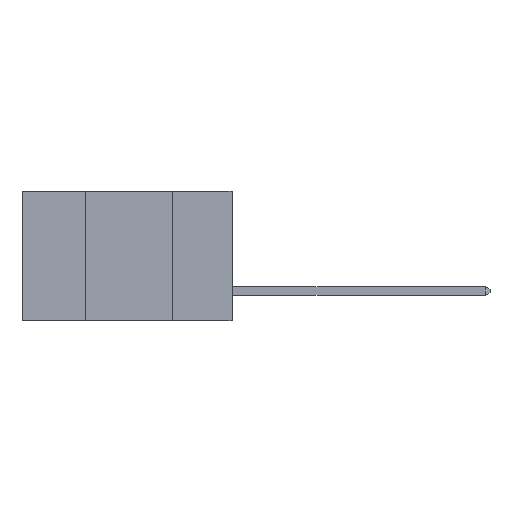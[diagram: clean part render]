
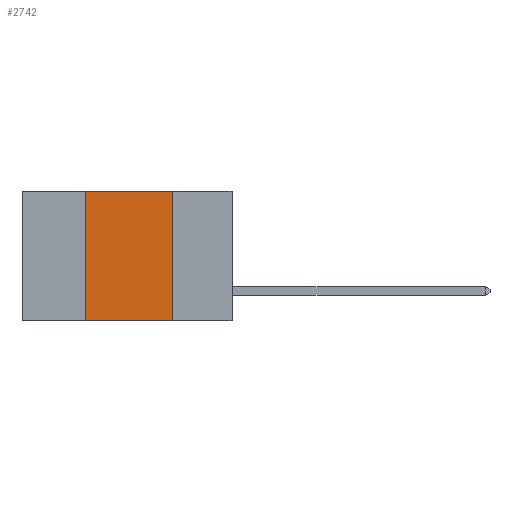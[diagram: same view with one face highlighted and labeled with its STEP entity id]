
A CAD part, left-side view. The second image highlights one B-rep face of the part: STEP entity #2742.
In plain terms, the highlighted planar face has unit normal (-1, 0, 0).
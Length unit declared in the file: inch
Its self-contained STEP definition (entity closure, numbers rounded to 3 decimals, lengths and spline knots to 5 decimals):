
#84 = DIRECTION ( 'NONE',  ( 0., -1., 0. ) ) ;
#383 = ORIENTED_EDGE ( 'NONE', *, *, #1739, .F. ) ;
#463 = VERTEX_POINT ( 'NONE', #9577 ) ;
#886 = VERTEX_POINT ( 'NONE', #2946 ) ;
#1046 = CARTESIAN_POINT ( 'NONE',  ( 0., 0.17, 0. ) ) ;
#1118 = DIRECTION ( 'NONE',  ( 0., 0., 1. ) ) ;
#1592 = AXIS2_PLACEMENT_3D ( 'NONE', #8293, #4157, #11375 ) ;
#1739 = EDGE_CURVE ( 'NONE', #463, #2903, #11052, .T. ) ;
#2147 = DIRECTION ( 'NONE',  ( 0., 0., -1. ) ) ;
#2742 = ADVANCED_FACE ( 'NONE', ( #7658 ), #12336, .F. ) ;
#2903 = VERTEX_POINT ( 'NONE', #6084 ) ;
#2946 = CARTESIAN_POINT ( 'NONE',  ( 0., 0.17, -0.37 ) ) ;
#3523 = CARTESIAN_POINT ( 'NONE',  ( 0., 0.42, -0.37 ) ) ;
#3797 = ORIENTED_EDGE ( 'NONE', *, *, #4467, .F. ) ;
#3812 = LINE ( 'NONE', #10682, #6924 ) ;
#4157 = DIRECTION ( 'NONE',  ( 1., 0., 0. ) ) ;
#4366 = CARTESIAN_POINT ( 'NONE',  ( 0., 0.42, 0. ) ) ;
#4467 = EDGE_CURVE ( 'NONE', #2903, #886, #12710, .T. ) ;
#5779 = DIRECTION ( 'NONE',  ( 0., -1., 0. ) ) ;
#5930 = EDGE_CURVE ( 'NONE', #6036, #886, #3812, .T. ) ;
#6036 = VERTEX_POINT ( 'NONE', #3523 ) ;
#6084 = CARTESIAN_POINT ( 'NONE',  ( 0., 0.17, 0. ) ) ;
#6924 = VECTOR ( 'NONE', #84, 39.37008 ) ;
#7294 = EDGE_LOOP ( 'NONE', ( #3797, #383, #13451, #9332 ) ) ;
#7658 = FACE_OUTER_BOUND ( 'NONE', #7294, .T. ) ;
#8064 = EDGE_CURVE ( 'NONE', #6036, #463, #11810, .T. ) ;
#8293 = CARTESIAN_POINT ( 'NONE',  ( 0., 0.6, 0. ) ) ;
#9090 = VECTOR ( 'NONE', #1118, 39.37008 ) ;
#9332 = ORIENTED_EDGE ( 'NONE', *, *, #5930, .T. ) ;
#9577 = CARTESIAN_POINT ( 'NONE',  ( 0., 0.42, 0. ) ) ;
#10024 = VECTOR ( 'NONE', #2147, 39.37008 ) ;
#10682 = CARTESIAN_POINT ( 'NONE',  ( 0., 0.6, -0.37 ) ) ;
#10732 = VECTOR ( 'NONE', #5779, 39.37008 ) ;
#11052 = LINE ( 'NONE', #12933, #10732 ) ;
#11375 = DIRECTION ( 'NONE',  ( 0., 0., -1. ) ) ;
#11810 = LINE ( 'NONE', #4366, #9090 ) ;
#12336 = PLANE ( 'NONE',  #1592 ) ;
#12710 = LINE ( 'NONE', #1046, #10024 ) ;
#12933 = CARTESIAN_POINT ( 'NONE',  ( 0., 0.6, 0. ) ) ;
#13451 = ORIENTED_EDGE ( 'NONE', *, *, #8064, .F. ) ;
